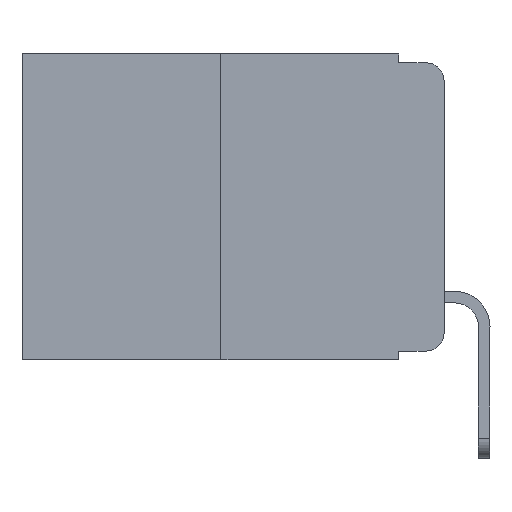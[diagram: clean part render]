
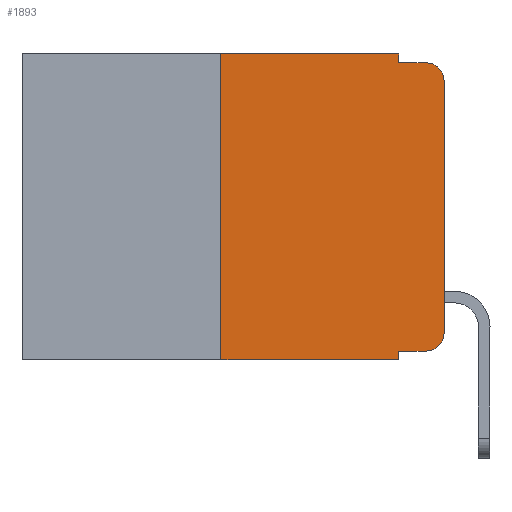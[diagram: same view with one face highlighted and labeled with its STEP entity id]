
A CAD part, left-side view. The second image highlights one B-rep face of the part: STEP entity #1893.
In plain terms, the highlighted planar face has unit normal (-1, 0, 0).
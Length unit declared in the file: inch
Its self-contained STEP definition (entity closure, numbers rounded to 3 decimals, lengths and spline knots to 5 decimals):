
#12 = VERTEX_POINT ( 'NONE', #5107 ) ;
#47 = CARTESIAN_POINT ( 'NONE',  ( 0., 0.25, 0. ) ) ;
#88 = LINE ( 'NONE', #6207, #4250 ) ;
#218 = CIRCLE ( 'NONE', #1146, 0.02 ) ;
#221 = CARTESIAN_POINT ( 'NONE',  ( 0., 0.051, -0.343 ) ) ;
#380 = CARTESIAN_POINT ( 'NONE',  ( 0., 0.02, -0.01 ) ) ;
#479 = LINE ( 'NONE', #2788, #8771 ) ;
#576 = DIRECTION ( 'NONE',  ( -1., 0., 0. ) ) ;
#686 = CARTESIAN_POINT ( 'NONE',  ( 0., 0.25, -0.343 ) ) ;
#735 = ORIENTED_EDGE ( 'NONE', *, *, #5808, .F. ) ;
#739 = DIRECTION ( 'NONE',  ( 0., -1., 0. ) ) ;
#1146 = AXIS2_PLACEMENT_3D ( 'NONE', #4116, #3231, #8814 ) ;
#1266 = CARTESIAN_POINT ( 'NONE',  ( 0., 0.473, 0. ) ) ;
#1406 = EDGE_CURVE ( 'NONE', #2779, #3335, #1672, .T. ) ;
#1608 = ORIENTED_EDGE ( 'NONE', *, *, #10998, .T. ) ;
#1672 = LINE ( 'NONE', #2619, #11460 ) ;
#1880 = DIRECTION ( 'NONE',  ( 0., 0., -1. ) ) ;
#1893 = ADVANCED_FACE ( 'NONE', ( #2120 ), #10393, .F. ) ;
#1964 = VERTEX_POINT ( 'NONE', #221 ) ;
#2059 = VERTEX_POINT ( 'NONE', #686 ) ;
#2120 = FACE_OUTER_BOUND ( 'NONE', #9658, .T. ) ;
#2160 = VECTOR ( 'NONE', #1880, 39.37008 ) ;
#2501 = CIRCLE ( 'NONE', #3600, 0.02 ) ;
#2543 = ORIENTED_EDGE ( 'NONE', *, *, #3606, .F. ) ;
#2619 = CARTESIAN_POINT ( 'NONE',  ( 0., 0., 0. ) ) ;
#2647 = CARTESIAN_POINT ( 'NONE',  ( 0., 0.051, -0.01 ) ) ;
#2779 = VERTEX_POINT ( 'NONE', #11152 ) ;
#2788 = CARTESIAN_POINT ( 'NONE',  ( 0., 0.051, -0.333 ) ) ;
#2923 = ORIENTED_EDGE ( 'NONE', *, *, #10995, .T. ) ;
#3172 = LINE ( 'NONE', #8163, #10040 ) ;
#3231 = DIRECTION ( 'NONE',  ( -1., 0., 0. ) ) ;
#3309 = ORIENTED_EDGE ( 'NONE', *, *, #10916, .F. ) ;
#3335 = VERTEX_POINT ( 'NONE', #11506 ) ;
#3348 = ORIENTED_EDGE ( 'NONE', *, *, #4479, .T. ) ;
#3385 = AXIS2_PLACEMENT_3D ( 'NONE', #1266, #9392, #7559 ) ;
#3517 = CARTESIAN_POINT ( 'NONE',  ( 0., 0.473, 0. ) ) ;
#3587 = VECTOR ( 'NONE', #10153, 39.37008 ) ;
#3600 = AXIS2_PLACEMENT_3D ( 'NONE', #6059, #576, #11501 ) ;
#3606 = EDGE_CURVE ( 'NONE', #2059, #11290, #4440, .T. ) ;
#3981 = ORIENTED_EDGE ( 'NONE', *, *, #8621, .F. ) ;
#4116 = CARTESIAN_POINT ( 'NONE',  ( 0., 0.02, -0.313 ) ) ;
#4250 = VECTOR ( 'NONE', #7297, 39.37008 ) ;
#4440 = LINE ( 'NONE', #47, #3587 ) ;
#4479 = EDGE_CURVE ( 'NONE', #2059, #1964, #4714, .T. ) ;
#4562 = CARTESIAN_POINT ( 'NONE',  ( 0., 0.051, 0. ) ) ;
#4714 = LINE ( 'NONE', #8659, #4864 ) ;
#4799 = LINE ( 'NONE', #3517, #7805 ) ;
#4864 = VECTOR ( 'NONE', #10510, 39.37008 ) ;
#5107 = CARTESIAN_POINT ( 'NONE',  ( 0., 0.051, 0. ) ) ;
#5116 = ORIENTED_EDGE ( 'NONE', *, *, #11872, .T. ) ;
#5524 = VERTEX_POINT ( 'NONE', #9661 ) ;
#5808 = EDGE_CURVE ( 'NONE', #5927, #6678, #88, .T. ) ;
#5927 = VERTEX_POINT ( 'NONE', #2647 ) ;
#6059 = CARTESIAN_POINT ( 'NONE',  ( 0., 0.02, -0.03 ) ) ;
#6207 = CARTESIAN_POINT ( 'NONE',  ( 0., 0.051, -0.01 ) ) ;
#6231 = CARTESIAN_POINT ( 'NONE',  ( 0., 0.25, 0. ) ) ;
#6345 = DIRECTION ( 'NONE',  ( 0., 0., -1. ) ) ;
#6678 = VERTEX_POINT ( 'NONE', #380 ) ;
#6799 = ORIENTED_EDGE ( 'NONE', *, *, #8506, .F. ) ;
#7104 = VERTEX_POINT ( 'NONE', #7293 ) ;
#7181 = DIRECTION ( 'NONE',  ( 0., -1., 0. ) ) ;
#7293 = CARTESIAN_POINT ( 'NONE',  ( 0., 0.02, -0.333 ) ) ;
#7297 = DIRECTION ( 'NONE',  ( 0., -1., 0. ) ) ;
#7559 = DIRECTION ( 'NONE',  ( 0., 0., -1. ) ) ;
#7805 = VECTOR ( 'NONE', #739, 39.37008 ) ;
#8163 = CARTESIAN_POINT ( 'NONE',  ( 0., 0.051, 0. ) ) ;
#8506 = EDGE_CURVE ( 'NONE', #12, #5927, #3172, .T. ) ;
#8621 = EDGE_CURVE ( 'NONE', #5524, #1964, #9463, .T. ) ;
#8659 = CARTESIAN_POINT ( 'NONE',  ( 0., 0.473, -0.343 ) ) ;
#8771 = VECTOR ( 'NONE', #7181, 39.37008 ) ;
#8814 = DIRECTION ( 'NONE',  ( 0., 0., -1. ) ) ;
#9392 = DIRECTION ( 'NONE',  ( 1., 0., 0. ) ) ;
#9463 = LINE ( 'NONE', #4562, #2160 ) ;
#9658 = EDGE_LOOP ( 'NONE', ( #11917, #1608, #735, #6799, #3309, #2543, #3348, #3981, #5116, #2923 ) ) ;
#9661 = CARTESIAN_POINT ( 'NONE',  ( 0., 0.051, -0.333 ) ) ;
#10037 = DIRECTION ( 'NONE',  ( 0., 0., 1. ) ) ;
#10040 = VECTOR ( 'NONE', #6345, 39.37008 ) ;
#10153 = DIRECTION ( 'NONE',  ( 0., 0., 1. ) ) ;
#10393 = PLANE ( 'NONE',  #3385 ) ;
#10510 = DIRECTION ( 'NONE',  ( 0., -1., 0. ) ) ;
#10916 = EDGE_CURVE ( 'NONE', #11290, #12, #4799, .T. ) ;
#10995 = EDGE_CURVE ( 'NONE', #7104, #2779, #218, .T. ) ;
#10998 = EDGE_CURVE ( 'NONE', #3335, #6678, #2501, .T. ) ;
#11152 = CARTESIAN_POINT ( 'NONE',  ( 0., 0., -0.313 ) ) ;
#11290 = VERTEX_POINT ( 'NONE', #6231 ) ;
#11460 = VECTOR ( 'NONE', #10037, 39.37008 ) ;
#11501 = DIRECTION ( 'NONE',  ( 0., 0., -1. ) ) ;
#11506 = CARTESIAN_POINT ( 'NONE',  ( 0., 0., -0.03 ) ) ;
#11872 = EDGE_CURVE ( 'NONE', #5524, #7104, #479, .T. ) ;
#11917 = ORIENTED_EDGE ( 'NONE', *, *, #1406, .T. ) ;
